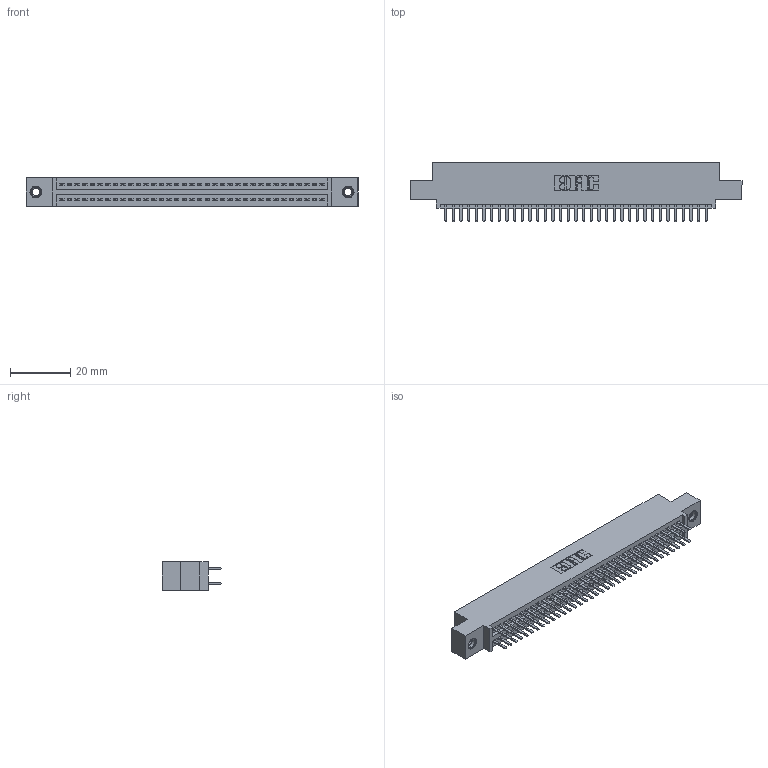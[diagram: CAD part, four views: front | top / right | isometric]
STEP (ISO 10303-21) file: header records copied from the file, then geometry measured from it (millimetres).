
FILE_DESCRIPTION (( 'STEP AP203' ), '1' );
FILE_NAME ('345-070-520-507.STEP', '2019-10-30T23:43:26', ( '' ), ( '' ), 'SwSTEP 2.0', 'SolidWorks 2016', '' );
FILE_SCHEMA (( 'CONFIG_CONTROL_DESIGN' ));
Length unit declared in the file: inch
Products named in the file (4): 345-292-001_345-293-120; 345 Part_0.110 Offset - 0.156 Dia-TI; 345-250-001_345-250-005-103; 345-070-520-507
Assembly tree (73 placements, depth 2):
  345-070-520-507
    345 Part_0.110 Offset - 0.156 Dia-TI
    345-292-001_345-293-120  x70
    345-250-001_345-250-005-103  x2
Bounding box: 110.11 x 19.68 x 9.4 mm (x, y, z)
Volume: 10513.5 mm3; surface area: 15460.4 mm2
Topology: 73 solids, 73 shells, 3970 faces, 11479 edges, 7458 vertices
Faces by surface type: plane 2566, cylinder 1388, cone 12, torus 4
Entity records: 29836 total; most frequent: CARTESIAN_POINT 5003, ORIENTED_EDGE 4918, DIRECTION 4433, EDGE_CURVE 2459, LINE 2163, VECTOR 2163, VERTEX_POINT 1632, AXIS2_PLACEMENT_3D 1135
